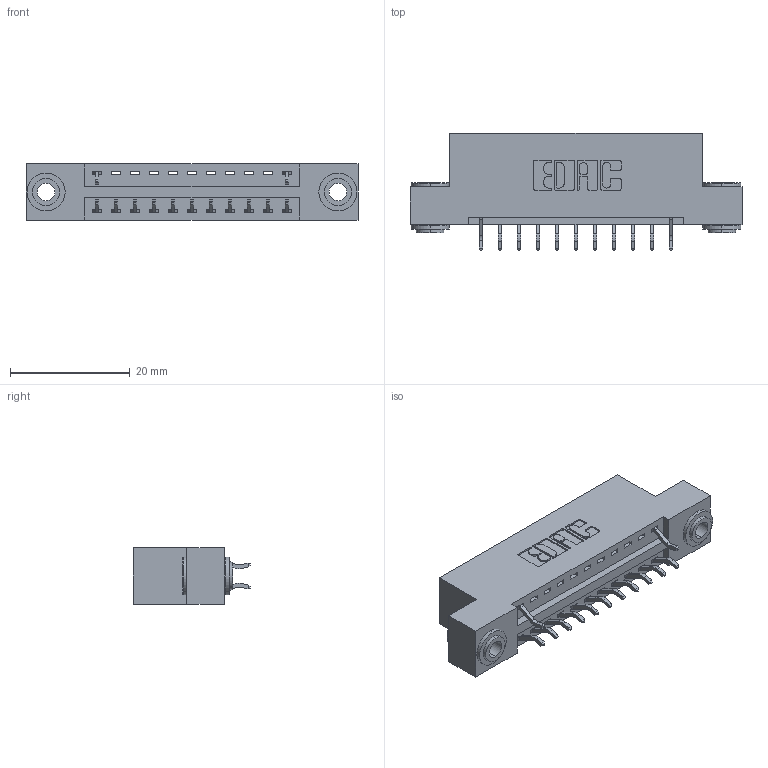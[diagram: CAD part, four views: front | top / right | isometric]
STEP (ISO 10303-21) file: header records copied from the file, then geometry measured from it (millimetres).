
FILE_DESCRIPTION (( 'STEP AP203' ), '1' );
FILE_NAME ('346-022-556-203.STEP', '2018-08-21T00:56:40', ( '' ), ( '' ), 'SwSTEP 2.0', 'SolidWorks 2016', '' );
FILE_SCHEMA (( 'CONFIG_CONTROL_DESIGN' ));
Length unit declared in the file: inch
Products named in the file (4): 346 Part_Flush Mounting Lugs - 0.156 Dia-TH; 345-292-001_556 Tail; 345-250-002_345-250-002-102; 346-022-556-203
Assembly tree (16 placements, depth 2):
  346-022-556-203
    346 Part_Flush Mounting Lugs - 0.156 Dia-TH
    345-292-001_556 Tail  x13
    345-250-002_345-250-002-102  x2
Bounding box: 55.5 x 19.57 x 9.4 mm (x, y, z)
Volume: 5109 mm3; surface area: 6270.4 mm2
Topology: 16 solids, 16 shells, 968 faces, 2843 edges, 1874 vertices
Faces by surface type: plane 638, cylinder 322, cone 8
Entity records: 11934 total; most frequent: CARTESIAN_POINT 2038, ORIENTED_EDGE 1962, DIRECTION 1857, EDGE_CURVE 981, VECTOR 773, LINE 773, VERTEX_POINT 650, AXIS2_PLACEMENT_3D 542
